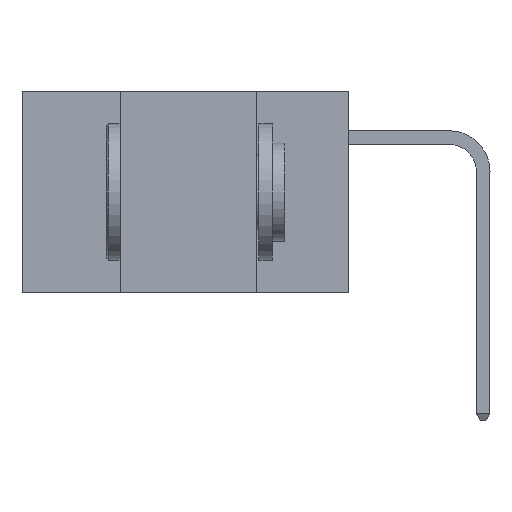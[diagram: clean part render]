
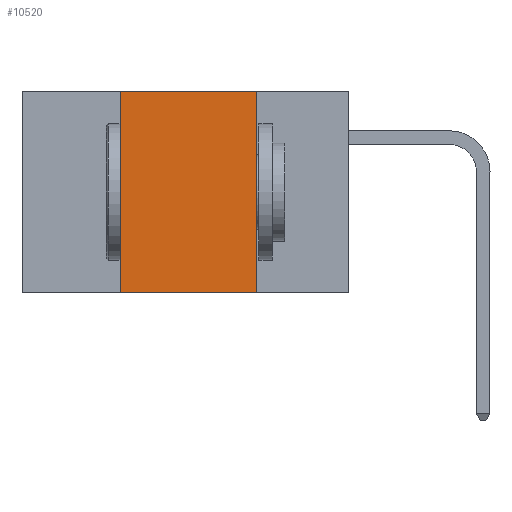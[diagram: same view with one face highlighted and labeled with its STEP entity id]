
A CAD part, left-side view. The second image highlights one B-rep face of the part: STEP entity #10520.
In plain terms, the highlighted planar face has unit normal (-1, 0, 0).
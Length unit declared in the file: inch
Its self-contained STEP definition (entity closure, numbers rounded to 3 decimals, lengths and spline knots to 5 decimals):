
#134 = VECTOR ( 'NONE', #4813, 39.37008 ) ;
#496 = VERTEX_POINT ( 'NONE', #6815 ) ;
#1013 = VECTOR ( 'NONE', #12157, 39.37008 ) ;
#1907 = EDGE_CURVE ( 'NONE', #3491, #4081, #10557, .T. ) ;
#2045 = CARTESIAN_POINT ( 'NONE',  ( 0., 0.6, 0. ) ) ;
#2263 = CARTESIAN_POINT ( 'NONE',  ( 0., 0.42, -0.37 ) ) ;
#2305 = DIRECTION ( 'NONE',  ( 0., 0., -1. ) ) ;
#3082 = DIRECTION ( 'NONE',  ( 1., 0., 0. ) ) ;
#3211 = CARTESIAN_POINT ( 'NONE',  ( 0., 0.17, 0. ) ) ;
#3283 = VECTOR ( 'NONE', #2305, 39.37008 ) ;
#3460 = ORIENTED_EDGE ( 'NONE', *, *, #12666, .F. ) ;
#3491 = VERTEX_POINT ( 'NONE', #2263 ) ;
#4081 = VERTEX_POINT ( 'NONE', #9006 ) ;
#4813 = DIRECTION ( 'NONE',  ( 0., -1., 0. ) ) ;
#5785 = FACE_OUTER_BOUND ( 'NONE', #5881, .T. ) ;
#5881 = EDGE_LOOP ( 'NONE', ( #3460, #8268, #9210, #11124 ) ) ;
#5894 = LINE ( 'NONE', #3211, #3283 ) ;
#5921 = PLANE ( 'NONE',  #8387 ) ;
#6080 = LINE ( 'NONE', #9119, #1013 ) ;
#6214 = LINE ( 'NONE', #8990, #8647 ) ;
#6815 = CARTESIAN_POINT ( 'NONE',  ( 0., 0.42, 0. ) ) ;
#7190 = CARTESIAN_POINT ( 'NONE',  ( 0., 0.17, 0. ) ) ;
#8268 = ORIENTED_EDGE ( 'NONE', *, *, #11364, .F. ) ;
#8387 = AXIS2_PLACEMENT_3D ( 'NONE', #2045, #3082, #9991 ) ;
#8647 = VECTOR ( 'NONE', #9389, 39.37008 ) ;
#8990 = CARTESIAN_POINT ( 'NONE',  ( 0., 0.42, 0. ) ) ;
#9006 = CARTESIAN_POINT ( 'NONE',  ( 0., 0.17, -0.37 ) ) ;
#9119 = CARTESIAN_POINT ( 'NONE',  ( 0., 0.6, 0. ) ) ;
#9210 = ORIENTED_EDGE ( 'NONE', *, *, #12194, .F. ) ;
#9277 = VERTEX_POINT ( 'NONE', #7190 ) ;
#9389 = DIRECTION ( 'NONE',  ( 0., 0., 1. ) ) ;
#9991 = DIRECTION ( 'NONE',  ( 0., 0., -1. ) ) ;
#10520 = ADVANCED_FACE ( 'NONE', ( #5785 ), #5921, .F. ) ;
#10557 = LINE ( 'NONE', #11539, #134 ) ;
#11124 = ORIENTED_EDGE ( 'NONE', *, *, #1907, .T. ) ;
#11364 = EDGE_CURVE ( 'NONE', #496, #9277, #6080, .T. ) ;
#11539 = CARTESIAN_POINT ( 'NONE',  ( 0., 0.6, -0.37 ) ) ;
#12157 = DIRECTION ( 'NONE',  ( 0., -1., 0. ) ) ;
#12194 = EDGE_CURVE ( 'NONE', #3491, #496, #6214, .T. ) ;
#12666 = EDGE_CURVE ( 'NONE', #9277, #4081, #5894, .T. ) ;
